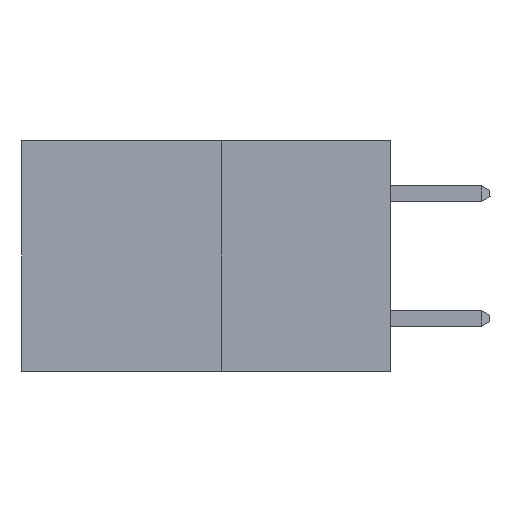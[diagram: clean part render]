
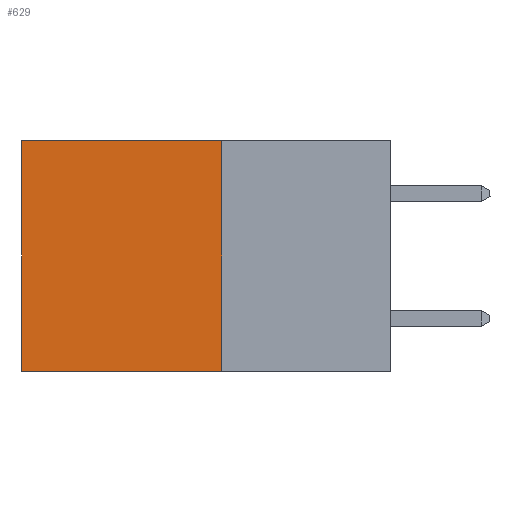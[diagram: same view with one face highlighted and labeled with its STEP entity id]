
A CAD part, left-side view. The second image highlights one B-rep face of the part: STEP entity #629.
In plain terms, the highlighted planar face has unit normal (-1, 0, 0).
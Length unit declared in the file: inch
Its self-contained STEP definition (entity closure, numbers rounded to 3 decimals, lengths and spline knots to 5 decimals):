
#267 = EDGE_LOOP ( 'NONE', ( #3570, #7728, #8208, #821 ) ) ;
#318 = LINE ( 'NONE', #7618, #12360 ) ;
#629 = ADVANCED_FACE ( 'NONE', ( #5887 ), #13531, .F. ) ;
#821 = ORIENTED_EDGE ( 'NONE', *, *, #14471, .T. ) ;
#929 = VERTEX_POINT ( 'NONE', #9734 ) ;
#2543 = DIRECTION ( 'NONE',  ( 0., 0., -1. ) ) ;
#3000 = CARTESIAN_POINT ( 'NONE',  ( 0.277, 0.27, -0.37 ) ) ;
#3270 = LINE ( 'NONE', #11931, #11612 ) ;
#3570 = ORIENTED_EDGE ( 'NONE', *, *, #18665, .T. ) ;
#3688 = EDGE_CURVE ( 'NONE', #3934, #7056, #318, .T. ) ;
#3934 = VERTEX_POINT ( 'NONE', #7396 ) ;
#4191 = DIRECTION ( 'NONE',  ( 0., 1., 0. ) ) ;
#4273 = VERTEX_POINT ( 'NONE', #19222 ) ;
#5887 = FACE_OUTER_BOUND ( 'NONE', #267, .T. ) ;
#7056 = VERTEX_POINT ( 'NONE', #3000 ) ;
#7396 = CARTESIAN_POINT ( 'NONE',  ( 0.277, 0.27, 0. ) ) ;
#7618 = CARTESIAN_POINT ( 'NONE',  ( 0.277, 0.27, -0.37 ) ) ;
#7728 = ORIENTED_EDGE ( 'NONE', *, *, #8158, .F. ) ;
#8158 = EDGE_CURVE ( 'NONE', #7056, #4273, #18838, .T. ) ;
#8208 = ORIENTED_EDGE ( 'NONE', *, *, #3688, .F. ) ;
#9734 = CARTESIAN_POINT ( 'NONE',  ( 0.277, 0.59, 0. ) ) ;
#11612 = VECTOR ( 'NONE', #2543, 39.37008 ) ;
#11931 = CARTESIAN_POINT ( 'NONE',  ( 0.277, 0.59, -0.37 ) ) ;
#12360 = VECTOR ( 'NONE', #19435, 39.37008 ) ;
#13154 = DIRECTION ( 'NONE',  ( 1., 0., 0. ) ) ;
#13221 = DIRECTION ( 'NONE',  ( 0., 0., -1. ) ) ;
#13311 = CARTESIAN_POINT ( 'NONE',  ( 0.277, 0.27, -0.37 ) ) ;
#13531 = PLANE ( 'NONE',  #19240 ) ;
#13867 = CARTESIAN_POINT ( 'NONE',  ( 0.277, 0.27, -0.37 ) ) ;
#14471 = EDGE_CURVE ( 'NONE', #3934, #929, #19129, .T. ) ;
#14750 = VECTOR ( 'NONE', #15275, 39.37008 ) ;
#14912 = VECTOR ( 'NONE', #4191, 39.37008 ) ;
#15275 = DIRECTION ( 'NONE',  ( 0., 1., 0. ) ) ;
#18197 = CARTESIAN_POINT ( 'NONE',  ( 0.277, 0.27, 0. ) ) ;
#18665 = EDGE_CURVE ( 'NONE', #929, #4273, #3270, .T. ) ;
#18838 = LINE ( 'NONE', #13867, #14912 ) ;
#19129 = LINE ( 'NONE', #18197, #14750 ) ;
#19222 = CARTESIAN_POINT ( 'NONE',  ( 0.277, 0.59, -0.37 ) ) ;
#19240 = AXIS2_PLACEMENT_3D ( 'NONE', #13311, #13154, #13221 ) ;
#19435 = DIRECTION ( 'NONE',  ( 0., 0., -1. ) ) ;
